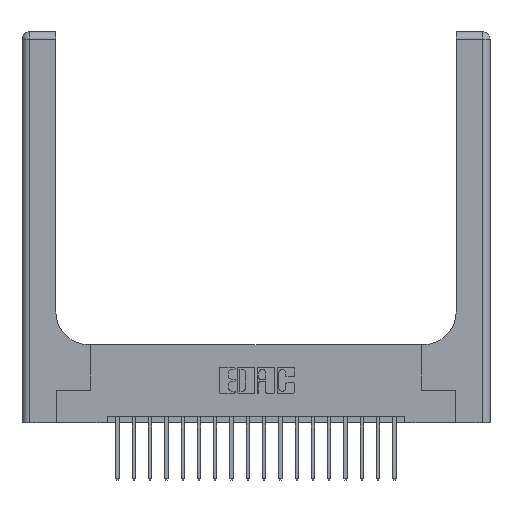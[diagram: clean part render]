
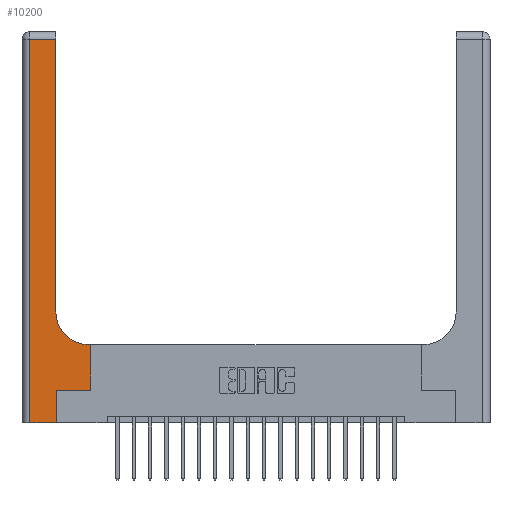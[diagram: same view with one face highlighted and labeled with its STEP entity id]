
A CAD part, top view. The second image highlights one B-rep face of the part: STEP entity #10200.
In plain terms, the highlighted planar face has unit normal (0, 0, 1).
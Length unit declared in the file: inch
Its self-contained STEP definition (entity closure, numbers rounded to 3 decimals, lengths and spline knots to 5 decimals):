
#156 = VECTOR ( 'NONE', #11740, 39.37008 ) ;
#166 = DIRECTION ( 'NONE',  ( 1., 0., 0. ) ) ;
#292 = CARTESIAN_POINT ( 'NONE',  ( 0.26, 0.85, 0.37 ) ) ;
#540 = LINE ( 'NONE', #1289, #15129 ) ;
#743 = DIRECTION ( 'NONE',  ( -1., 0., 0. ) ) ;
#1053 = ORIENTED_EDGE ( 'NONE', *, *, #9137, .T. ) ;
#1177 = VERTEX_POINT ( 'NONE', #19331 ) ;
#1289 = CARTESIAN_POINT ( 'NONE',  ( 0.26, 3., 0.37 ) ) ;
#1640 = EDGE_CURVE ( 'NONE', #3864, #15426, #15385, .T. ) ;
#1933 = VECTOR ( 'NONE', #18477, 39.37008 ) ;
#2294 = CARTESIAN_POINT ( 'NONE',  ( 0.51, 0.6, 0.37 ) ) ;
#2524 = FACE_OUTER_BOUND ( 'NONE', #3015, .T. ) ;
#3015 = EDGE_LOOP ( 'NONE', ( #8203, #4655, #4795, #16539, #8548, #19759, #7082, #17826, #1053 ) ) ;
#3523 = CARTESIAN_POINT ( 'NONE',  ( 0.528, 0.6, 0.37 ) ) ;
#3611 = VECTOR ( 'NONE', #13470, 39.37008 ) ;
#3864 = VERTEX_POINT ( 'NONE', #17622 ) ;
#4075 = CARTESIAN_POINT ( 'NONE',  ( 0.51, 0.85, 0.37 ) ) ;
#4603 = CARTESIAN_POINT ( 'NONE',  ( 0.528, 0.25, 0.37 ) ) ;
#4655 = ORIENTED_EDGE ( 'NONE', *, *, #13651, .T. ) ;
#4758 = VERTEX_POINT ( 'NONE', #6988 ) ;
#4795 = ORIENTED_EDGE ( 'NONE', *, *, #14287, .T. ) ;
#5378 = VECTOR ( 'NONE', #5960, 39.37008 ) ;
#5960 = DIRECTION ( 'NONE',  ( 0., 1., 0. ) ) ;
#6006 = LINE ( 'NONE', #8837, #156 ) ;
#6021 = VERTEX_POINT ( 'NONE', #3523 ) ;
#6086 = LINE ( 'NONE', #4603, #1933 ) ;
#6177 = DIRECTION ( 'NONE',  ( 0., 1., 0. ) ) ;
#6207 = CIRCLE ( 'NONE', #17015, 0.25 ) ;
#6719 = EDGE_CURVE ( 'NONE', #6021, #17806, #9445, .T. ) ;
#6836 = CARTESIAN_POINT ( 'NONE',  ( 0.26, 2.94, 0.37 ) ) ;
#6988 = CARTESIAN_POINT ( 'NONE',  ( 0.06, 0., 0.37 ) ) ;
#7082 = ORIENTED_EDGE ( 'NONE', *, *, #12533, .T. ) ;
#7585 = VERTEX_POINT ( 'NONE', #9381 ) ;
#7595 = DIRECTION ( 'NONE',  ( -1., 0., 0. ) ) ;
#7762 = LINE ( 'NONE', #13202, #3611 ) ;
#8079 = VECTOR ( 'NONE', #166, 39.37008 ) ;
#8203 = ORIENTED_EDGE ( 'NONE', *, *, #16422, .T. ) ;
#8548 = ORIENTED_EDGE ( 'NONE', *, *, #11121, .T. ) ;
#8837 = CARTESIAN_POINT ( 'NONE',  ( 0.06, 3., 0.37 ) ) ;
#9137 = EDGE_CURVE ( 'NONE', #17806, #17091, #6207, .T. ) ;
#9381 = CARTESIAN_POINT ( 'NONE',  ( 0.06, 2.94, 0.37 ) ) ;
#9445 = LINE ( 'NONE', #13949, #15248 ) ;
#9486 = CARTESIAN_POINT ( 'NONE',  ( 0.265, 0.25, 0.37 ) ) ;
#10200 = ADVANCED_FACE ( 'NONE', ( #2524 ), #14674, .F. ) ;
#10466 = EDGE_CURVE ( 'NONE', #4758, #1177, #17525, .T. ) ;
#10614 = CARTESIAN_POINT ( 'NONE',  ( 0.265, 0., 0.37 ) ) ;
#10672 = DIRECTION ( 'NONE',  ( 0., 0., -1. ) ) ;
#11121 = EDGE_CURVE ( 'NONE', #1177, #3864, #14357, .T. ) ;
#11567 = AXIS2_PLACEMENT_3D ( 'NONE', #19401, #11642, #743 ) ;
#11642 = DIRECTION ( 'NONE',  ( 0., 0., -1. ) ) ;
#11740 = DIRECTION ( 'NONE',  ( 0., -1., 0. ) ) ;
#12279 = VECTOR ( 'NONE', #13982, 39.37008 ) ;
#12533 = EDGE_CURVE ( 'NONE', #15426, #6021, #6086, .T. ) ;
#13202 = CARTESIAN_POINT ( 'NONE',  ( 0., 2.94, 0.37 ) ) ;
#13470 = DIRECTION ( 'NONE',  ( -1., 0., 0. ) ) ;
#13578 = DIRECTION ( 'NONE',  ( 1., 0., 0. ) ) ;
#13651 = EDGE_CURVE ( 'NONE', #15063, #7585, #7762, .T. ) ;
#13949 = CARTESIAN_POINT ( 'NONE',  ( 0.26, 0.6, 0.37 ) ) ;
#13982 = DIRECTION ( 'NONE',  ( 1., 0., 0. ) ) ;
#14287 = EDGE_CURVE ( 'NONE', #7585, #4758, #6006, .T. ) ;
#14357 = LINE ( 'NONE', #10614, #5378 ) ;
#14674 = PLANE ( 'NONE',  #11567 ) ;
#15063 = VERTEX_POINT ( 'NONE', #6836 ) ;
#15129 = VECTOR ( 'NONE', #6177, 39.37008 ) ;
#15248 = VECTOR ( 'NONE', #7595, 39.37008 ) ;
#15385 = LINE ( 'NONE', #9486, #12279 ) ;
#15426 = VERTEX_POINT ( 'NONE', #15710 ) ;
#15710 = CARTESIAN_POINT ( 'NONE',  ( 0.528, 0.25, 0.37 ) ) ;
#16422 = EDGE_CURVE ( 'NONE', #17091, #15063, #540, .T. ) ;
#16539 = ORIENTED_EDGE ( 'NONE', *, *, #10466, .T. ) ;
#17015 = AXIS2_PLACEMENT_3D ( 'NONE', #4075, #10672, #13578 ) ;
#17091 = VERTEX_POINT ( 'NONE', #292 ) ;
#17525 = LINE ( 'NONE', #18487, #8079 ) ;
#17622 = CARTESIAN_POINT ( 'NONE',  ( 0.265, 0.25, 0.37 ) ) ;
#17806 = VERTEX_POINT ( 'NONE', #2294 ) ;
#17826 = ORIENTED_EDGE ( 'NONE', *, *, #6719, .T. ) ;
#18477 = DIRECTION ( 'NONE',  ( 0., 1., 0. ) ) ;
#18487 = CARTESIAN_POINT ( 'NONE',  ( 0., 0., 0.37 ) ) ;
#19331 = CARTESIAN_POINT ( 'NONE',  ( 0.265, 0., 0.37 ) ) ;
#19401 = CARTESIAN_POINT ( 'NONE',  ( 0., 3., 0.37 ) ) ;
#19759 = ORIENTED_EDGE ( 'NONE', *, *, #1640, .T. ) ;
